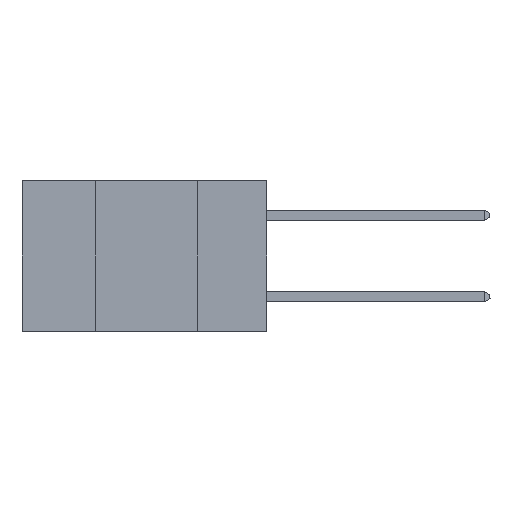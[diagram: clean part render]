
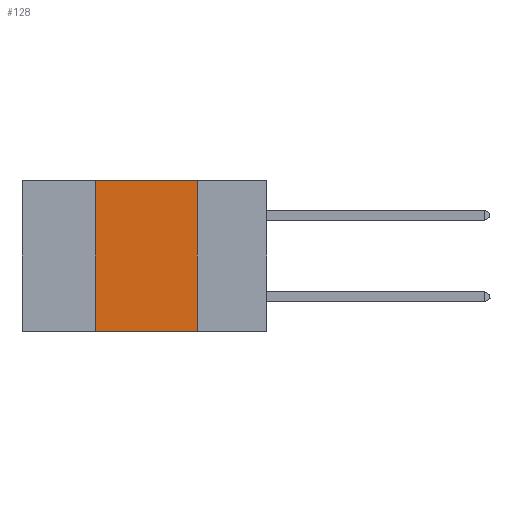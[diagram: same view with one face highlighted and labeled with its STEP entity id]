
A CAD part, left-side view. The second image highlights one B-rep face of the part: STEP entity #128.
In plain terms, the highlighted planar face has unit normal (-1, 0, 0).
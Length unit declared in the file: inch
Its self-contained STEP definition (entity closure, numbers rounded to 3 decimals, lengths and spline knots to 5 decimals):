
#128 = ADVANCED_FACE ( 'NONE', ( #9475 ), #10449, .F. ) ;
#3190 = LINE ( 'NONE', #11704, #20639 ) ;
#4129 = DIRECTION ( 'NONE',  ( 0., 0., -1. ) ) ;
#4202 = DIRECTION ( 'NONE',  ( 1., 0., 0. ) ) ;
#4873 = EDGE_CURVE ( 'NONE', #20649, #19233, #3190, .T. ) ;
#5688 = LINE ( 'NONE', #5782, #14430 ) ;
#5782 = CARTESIAN_POINT ( 'NONE',  ( 0., 0.42, 0. ) ) ;
#5788 = ORIENTED_EDGE ( 'NONE', *, *, #4873, .F. ) ;
#7523 = DIRECTION ( 'NONE',  ( 0., 0., 1. ) ) ;
#8005 = CARTESIAN_POINT ( 'NONE',  ( 0., 0.17, 0. ) ) ;
#9306 = ORIENTED_EDGE ( 'NONE', *, *, #21187, .F. ) ;
#9475 = FACE_OUTER_BOUND ( 'NONE', #14235, .T. ) ;
#9629 = DIRECTION ( 'NONE',  ( 0., -1., 0. ) ) ;
#10119 = CARTESIAN_POINT ( 'NONE',  ( 0., 0.42, -0.37 ) ) ;
#10449 = PLANE ( 'NONE',  #17874 ) ;
#10559 = CARTESIAN_POINT ( 'NONE',  ( 0., 0.6, 0. ) ) ;
#11704 = CARTESIAN_POINT ( 'NONE',  ( 0., 0.6, 0. ) ) ;
#12245 = VECTOR ( 'NONE', #18392, 39.37008 ) ;
#13433 = DIRECTION ( 'NONE',  ( 0., -1., 0. ) ) ;
#14235 = EDGE_LOOP ( 'NONE', ( #9306, #5788, #15045, #15589 ) ) ;
#14430 = VECTOR ( 'NONE', #7523, 39.37008 ) ;
#15045 = ORIENTED_EDGE ( 'NONE', *, *, #22168, .F. ) ;
#15335 = EDGE_CURVE ( 'NONE', #19982, #19872, #19956, .T. ) ;
#15589 = ORIENTED_EDGE ( 'NONE', *, *, #15335, .T. ) ;
#15967 = VECTOR ( 'NONE', #9629, 39.37008 ) ;
#16697 = CARTESIAN_POINT ( 'NONE',  ( 0., 0.17, 0. ) ) ;
#17012 = CARTESIAN_POINT ( 'NONE',  ( 0., 0.42, 0. ) ) ;
#17825 = LINE ( 'NONE', #16697, #12245 ) ;
#17874 = AXIS2_PLACEMENT_3D ( 'NONE', #10559, #4202, #4129 ) ;
#18392 = DIRECTION ( 'NONE',  ( 0., 0., -1. ) ) ;
#19233 = VERTEX_POINT ( 'NONE', #8005 ) ;
#19872 = VERTEX_POINT ( 'NONE', #21754 ) ;
#19956 = LINE ( 'NONE', #19963, #15967 ) ;
#19963 = CARTESIAN_POINT ( 'NONE',  ( 0., 0.6, -0.37 ) ) ;
#19982 = VERTEX_POINT ( 'NONE', #10119 ) ;
#20639 = VECTOR ( 'NONE', #13433, 39.37008 ) ;
#20649 = VERTEX_POINT ( 'NONE', #17012 ) ;
#21187 = EDGE_CURVE ( 'NONE', #19233, #19872, #17825, .T. ) ;
#21754 = CARTESIAN_POINT ( 'NONE',  ( 0., 0.17, -0.37 ) ) ;
#22168 = EDGE_CURVE ( 'NONE', #19982, #20649, #5688, .T. ) ;
